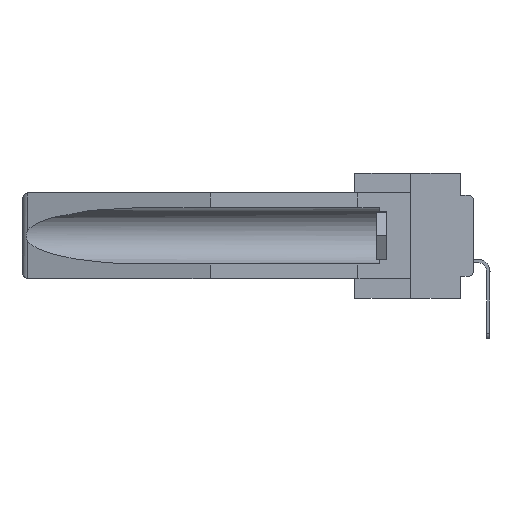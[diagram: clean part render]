
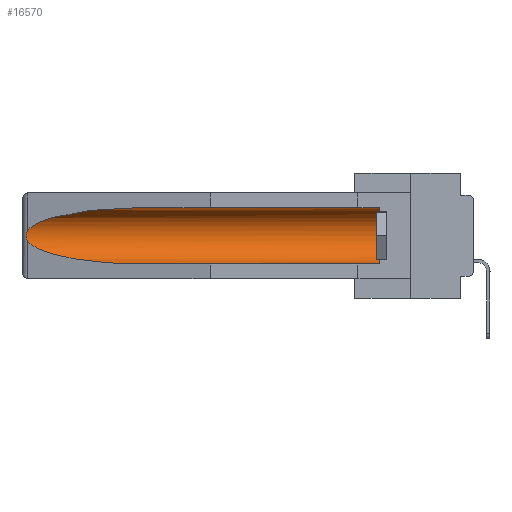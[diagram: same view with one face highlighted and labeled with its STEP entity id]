
A CAD part, left-side view. The second image highlights one B-rep face of the part: STEP entity #16570.
In plain terms, the highlighted cylindrical face has radius 2.857 mm (diameter 5.715 mm), a partial arc.
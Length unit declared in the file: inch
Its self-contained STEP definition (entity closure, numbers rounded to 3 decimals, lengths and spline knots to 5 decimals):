
#316 = VECTOR ( 'NONE', #18033, 39.37008 ) ;
#479 = CARTESIAN_POINT ( 'NONE',  ( 0.26655, 1.53094, -0.18657 ) ) ;
#1957 = AXIS2_PLACEMENT_3D ( 'NONE', #13493, #21460, #16362 ) ;
#3933 = CARTESIAN_POINT ( 'NONE',  ( 0.21114, 1.30732, -0.284 ) ) ;
#3951 = ORIENTED_EDGE ( 'NONE', *, *, #29107, .T. ) ;
#4889 = CARTESIAN_POINT ( 'NONE',  ( 0.26654, 1.53092, -0.15636 ) ) ;
#5436 = FACE_OUTER_BOUND ( 'NONE', #28730, .T. ) ;
#5587 = CARTESIAN_POINT ( 'NONE',  ( 0.26537, 1.52718, -0.14972 ) ) ;
#5659 = VERTEX_POINT ( 'NONE', #9271 ) ;
#6233 = ORIENTED_EDGE ( 'NONE', *, *, #21989, .T. ) ;
#7210 = CARTESIAN_POINT ( 'NONE',  ( 0.155, 0.126, -0.059 ) ) ;
#7735 = LINE ( 'NONE', #13279, #316 ) ;
#8571 = LINE ( 'NONE', #10416, #10350 ) ;
#9271 = CARTESIAN_POINT ( 'NONE',  ( 0.26537, 1.52718, -0.19328 ) ) ;
#10271 = EDGE_CURVE ( 'NONE', #31646, #17251, #8571, .T. ) ;
#10350 = VECTOR ( 'NONE', #20895, 39.37008 ) ;
#10354 = CYLINDRICAL_SURFACE ( 'NONE', #24957, 0.1125 ) ;
#10416 = CARTESIAN_POINT ( 'NONE',  ( 0.155, -0.30754, -0.284 ) ) ;
#10467 = CARTESIAN_POINT ( 'NONE',  ( 0.2673, 1.5327, -0.16383 ) ) ;
#10555 = CARTESIAN_POINT ( 'NONE',  ( 0.26537, 1.52718, -0.19328 ) ) ;
#10637 = CARTESIAN_POINT ( 'NONE',  ( 0.26597, 1.5296, -0.19026 ) ) ;
#10853 = DIRECTION ( 'NONE',  ( 0., 0., 1. ) ) ;
#11730 =( BOUNDED_CURVE ( )  B_SPLINE_CURVE ( 3, ( #10555, #31195, #3933, #29989 ),
 .UNSPECIFIED., .F., .T. ) 
 B_SPLINE_CURVE_WITH_KNOTS ( ( 4, 4 ),
 ( 0.1948, 1.5708 ),
 .UNSPECIFIED. ) 
 CURVE ( )  GEOMETRIC_REPRESENTATION_ITEM ( )  RATIONAL_B_SPLINE_CURVE ( ( 1., 0.848, 0.848, 1. ) ) 
 REPRESENTATION_ITEM ( '' )  );
#12026 = CARTESIAN_POINT ( 'NONE',  ( 0.25451, 1.48313, -0.09465 ) ) ;
#12626 = EDGE_CURVE ( 'NONE', #23968, #14928, #7735, .T. ) ;
#13279 = CARTESIAN_POINT ( 'NONE',  ( 0.155, -0.30754, -0.059 ) ) ;
#13493 = CARTESIAN_POINT ( 'NONE',  ( 0.155, 0.126, -0.1715 ) ) ;
#14928 = VERTEX_POINT ( 'NONE', #24543 ) ;
#15200 = CARTESIAN_POINT ( 'NONE',  ( 0.26537, 1.52718, -0.14972 ) ) ;
#15531 = CARTESIAN_POINT ( 'NONE',  ( 0.2675, 1.53308, -0.16763 ) ) ;
#16362 = DIRECTION ( 'NONE',  ( 0., 0., 1. ) ) ;
#16570 = ADVANCED_FACE ( 'NONE', ( #5436 ), #10354, .F. ) ;
#16825 = EDGE_CURVE ( 'NONE', #14928, #20407, #21021, .T. ) ;
#17251 = VERTEX_POINT ( 'NONE', #30707 ) ;
#17264 = CARTESIAN_POINT ( 'NONE',  ( 0.21114, 1.30732, -0.059 ) ) ;
#17483 = EDGE_CURVE ( 'NONE', #5659, #17251, #11730, .T. ) ;
#17757 = CARTESIAN_POINT ( 'NONE',  ( 0.155, 1.07973, -0.059 ) ) ;
#18033 = DIRECTION ( 'NONE',  ( 0., 1., 0. ) ) ;
#20407 = VERTEX_POINT ( 'NONE', #5587 ) ;
#20625 = CARTESIAN_POINT ( 'NONE',  ( 0.26597, 1.52961, -0.15275 ) ) ;
#20782 = CARTESIAN_POINT ( 'NONE',  ( 0.26537, 1.52718, -0.19328 ) ) ;
#20895 = DIRECTION ( 'NONE',  ( 0., 1., 0. ) ) ;
#21021 =( BOUNDED_CURVE ( )  B_SPLINE_CURVE ( 3, ( #17757, #17264, #12026, #27590 ),
 .UNSPECIFIED., .F., .F. ) 
 B_SPLINE_CURVE_WITH_KNOTS ( ( 4, 4 ),
 ( 4.71239, 6.08839 ),
 .UNSPECIFIED. ) 
 CURVE ( )  GEOMETRIC_REPRESENTATION_ITEM ( )  RATIONAL_B_SPLINE_CURVE ( ( 1., 0.848, 0.848, 1. ) ) 
 REPRESENTATION_ITEM ( '' )  );
#21460 = DIRECTION ( 'NONE',  ( 0., -1., 0. ) ) ;
#21989 = EDGE_CURVE ( 'NONE', #20407, #5659, #22927, .T. ) ;
#22927 = B_SPLINE_CURVE_WITH_KNOTS ( 'NONE', 3,
 ( #15200, #20625, #4889, #10467, #15531, #31262, #25868, #479, #10637, #20782 ),
 .UNSPECIFIED., .F., .F.,
 ( 4, 2, 2, 2, 4 ),
 ( 0., 0.00029, 0.00058, 0.00087, 0.00117 ),
 .UNSPECIFIED. ) ;
#23537 = DIRECTION ( 'NONE',  ( 0., 1., 0. ) ) ;
#23968 = VERTEX_POINT ( 'NONE', #7210 ) ;
#24543 = CARTESIAN_POINT ( 'NONE',  ( 0.155, 1.07973, -0.059 ) ) ;
#24957 = AXIS2_PLACEMENT_3D ( 'NONE', #31652, #23537, #10853 ) ;
#25868 = CARTESIAN_POINT ( 'NONE',  ( 0.2673, 1.53269, -0.17917 ) ) ;
#26250 = CIRCLE ( 'NONE', #1957, 0.1125 ) ;
#26771 = ORIENTED_EDGE ( 'NONE', *, *, #12626, .T. ) ;
#27590 = CARTESIAN_POINT ( 'NONE',  ( 0.26537, 1.52718, -0.14972 ) ) ;
#28730 = EDGE_LOOP ( 'NONE', ( #31055, #6233, #30163, #30644, #3951, #26771 ) ) ;
#29107 = EDGE_CURVE ( 'NONE', #31646, #23968, #26250, .T. ) ;
#29123 = CARTESIAN_POINT ( 'NONE',  ( 0.155, 0.126, -0.284 ) ) ;
#29989 = CARTESIAN_POINT ( 'NONE',  ( 0.155, 1.07973, -0.284 ) ) ;
#30163 = ORIENTED_EDGE ( 'NONE', *, *, #17483, .T. ) ;
#30644 = ORIENTED_EDGE ( 'NONE', *, *, #10271, .F. ) ;
#30707 = CARTESIAN_POINT ( 'NONE',  ( 0.155, 1.07973, -0.284 ) ) ;
#31055 = ORIENTED_EDGE ( 'NONE', *, *, #16825, .T. ) ;
#31195 = CARTESIAN_POINT ( 'NONE',  ( 0.25451, 1.48313, -0.24835 ) ) ;
#31262 = CARTESIAN_POINT ( 'NONE',  ( 0.2675, 1.53308, -0.17534 ) ) ;
#31646 = VERTEX_POINT ( 'NONE', #29123 ) ;
#31652 = CARTESIAN_POINT ( 'NONE',  ( 0.155, -0.30754, -0.1715 ) ) ;
